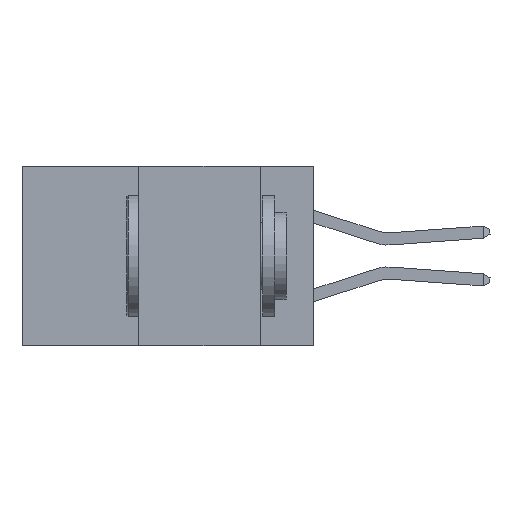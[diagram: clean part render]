
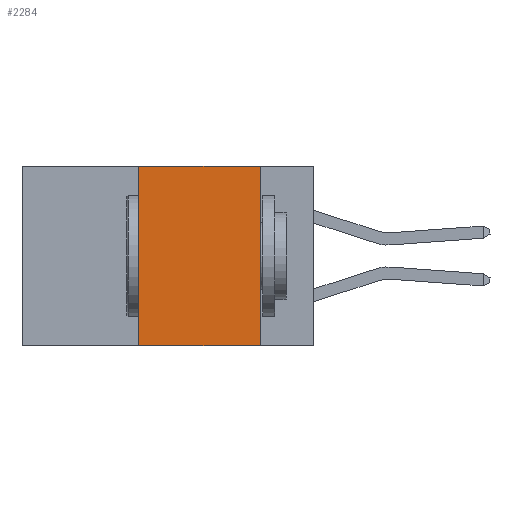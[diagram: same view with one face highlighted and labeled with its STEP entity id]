
A CAD part, left-side view. The second image highlights one B-rep face of the part: STEP entity #2284.
In plain terms, the highlighted planar face has unit normal (-1, 0, 0).
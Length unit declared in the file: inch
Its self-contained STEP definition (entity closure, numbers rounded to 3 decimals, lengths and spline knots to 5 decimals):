
#287 = VERTEX_POINT ( 'NONE', #9169 ) ;
#670 = VECTOR ( 'NONE', #20565, 39.37008 ) ;
#1640 = ORIENTED_EDGE ( 'NONE', *, *, #19119, .F. ) ;
#1949 = VECTOR ( 'NONE', #24538, 39.37008 ) ;
#2284 = ADVANCED_FACE ( 'NONE', ( #28863 ), #6154, .F. ) ;
#3199 = AXIS2_PLACEMENT_3D ( 'NONE', #17692, #15805, #31833 ) ;
#3254 = VECTOR ( 'NONE', #20612, 39.37008 ) ;
#3499 = VERTEX_POINT ( 'NONE', #13045 ) ;
#4219 = CARTESIAN_POINT ( 'NONE',  ( 0., 0.11, 0. ) ) ;
#4788 = DIRECTION ( 'NONE',  ( 0., -1., 0. ) ) ;
#6154 = PLANE ( 'NONE',  #3199 ) ;
#6353 = EDGE_CURVE ( 'NONE', #287, #13945, #25316, .T. ) ;
#7197 = VERTEX_POINT ( 'NONE', #12605 ) ;
#7456 = LINE ( 'NONE', #23374, #670 ) ;
#9169 = CARTESIAN_POINT ( 'NONE',  ( 0., 0.36, 0. ) ) ;
#9743 = EDGE_CURVE ( 'NONE', #3499, #7197, #27776, .T. ) ;
#9750 = CARTESIAN_POINT ( 'NONE',  ( 0., 0.6, 0. ) ) ;
#12605 = CARTESIAN_POINT ( 'NONE',  ( 0., 0.11, -0.37 ) ) ;
#13045 = CARTESIAN_POINT ( 'NONE',  ( 0., 0.36, -0.37 ) ) ;
#13257 = VECTOR ( 'NONE', #4788, 39.37008 ) ;
#13336 = EDGE_CURVE ( 'NONE', #3499, #287, #7456, .T. ) ;
#13945 = VERTEX_POINT ( 'NONE', #30192 ) ;
#14331 = LINE ( 'NONE', #4219, #1949 ) ;
#14509 = ORIENTED_EDGE ( 'NONE', *, *, #13336, .F. ) ;
#15692 = ORIENTED_EDGE ( 'NONE', *, *, #6353, .F. ) ;
#15805 = DIRECTION ( 'NONE',  ( 1., 0., 0. ) ) ;
#17692 = CARTESIAN_POINT ( 'NONE',  ( 0., 0.6, 0. ) ) ;
#19119 = EDGE_CURVE ( 'NONE', #13945, #7197, #14331, .T. ) ;
#20159 = CARTESIAN_POINT ( 'NONE',  ( 0., 0.6, -0.37 ) ) ;
#20565 = DIRECTION ( 'NONE',  ( 0., 0., 1. ) ) ;
#20612 = DIRECTION ( 'NONE',  ( 0., -1., 0. ) ) ;
#23374 = CARTESIAN_POINT ( 'NONE',  ( 0., 0.36, 0. ) ) ;
#23518 = EDGE_LOOP ( 'NONE', ( #1640, #15692, #14509, #30058 ) ) ;
#24538 = DIRECTION ( 'NONE',  ( 0., 0., -1. ) ) ;
#25316 = LINE ( 'NONE', #9750, #13257 ) ;
#27776 = LINE ( 'NONE', #20159, #3254 ) ;
#28863 = FACE_OUTER_BOUND ( 'NONE', #23518, .T. ) ;
#30058 = ORIENTED_EDGE ( 'NONE', *, *, #9743, .T. ) ;
#30192 = CARTESIAN_POINT ( 'NONE',  ( 0., 0.11, 0. ) ) ;
#31833 = DIRECTION ( 'NONE',  ( 0., 0., -1. ) ) ;
